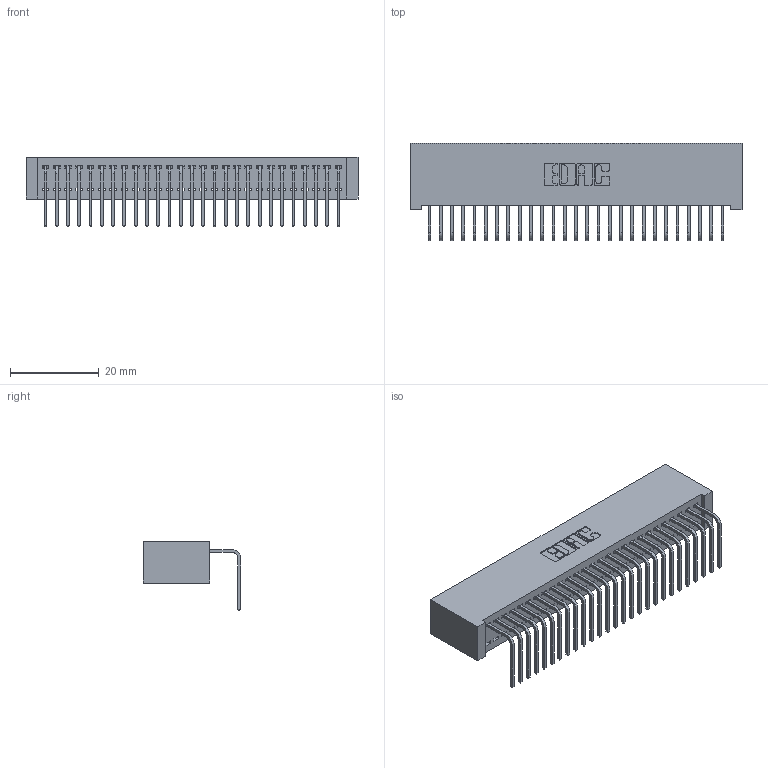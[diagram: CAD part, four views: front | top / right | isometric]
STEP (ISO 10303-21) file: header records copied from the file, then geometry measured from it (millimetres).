
FILE_DESCRIPTION (( 'STEP AP203' ), '1' );
FILE_NAME ('342-027-558-101.STEP', '2019-10-02T02:18:44', ( '' ), ( '' ), 'SwSTEP 2.0', 'SolidWorks 2016', '' );
FILE_SCHEMA (( 'CONFIG_CONTROL_DESIGN' ));
Length unit declared in the file: inch
Products named in the file (3): 342 Part_Lugless; 345-292-001_558 Tail - 2; 342-027-558-101
Assembly tree (28 placements, depth 2):
  342-027-558-101
    342 Part_Lugless
    345-292-001_558 Tail - 2  x27
Bounding box: 74.83 x 21.91 x 15.62 mm (x, y, z)
Volume: 7004.6 mm3; surface area: 10840.1 mm2
Topology: 28 solids, 28 shells, 1722 faces, 5189 edges, 3422 vertices
Faces by surface type: plane 1250, cylinder 472
Entity records: 18121 total; most frequent: CARTESIAN_POINT 3135, ORIENTED_EDGE 3098, DIRECTION 2667, EDGE_CURVE 1549, VECTOR 1429, LINE 1429, VERTEX_POINT 1030, AXIS2_PLACEMENT_3D 619
